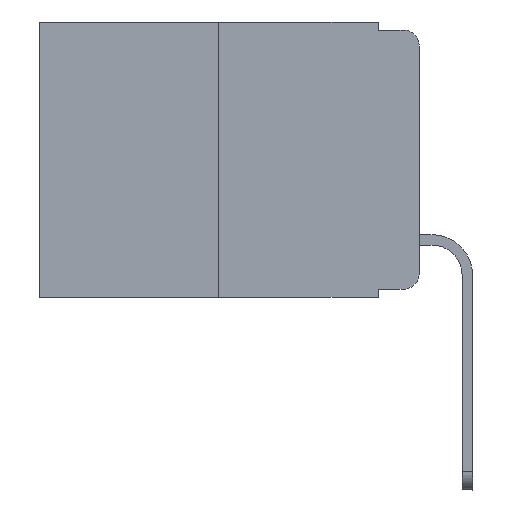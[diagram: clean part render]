
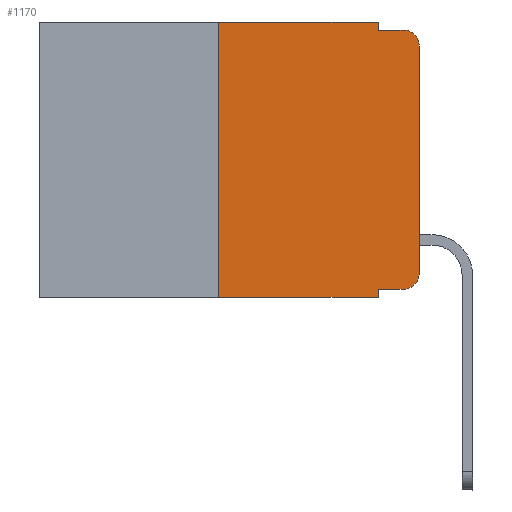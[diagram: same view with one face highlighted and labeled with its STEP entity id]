
A CAD part, left-side view. The second image highlights one B-rep face of the part: STEP entity #1170.
In plain terms, the highlighted planar face has unit normal (-1, 0, 0).
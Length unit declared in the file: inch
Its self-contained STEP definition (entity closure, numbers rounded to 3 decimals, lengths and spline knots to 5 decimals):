
#82 = EDGE_CURVE ( 'NONE', #13693, #13190, #6602, .T. ) ;
#115 = CARTESIAN_POINT ( 'NONE',  ( 0., 0.02, -0.333 ) ) ;
#317 = DIRECTION ( 'NONE',  ( 0., 0., -1. ) ) ;
#333 = DIRECTION ( 'NONE',  ( 0., -1., 0. ) ) ;
#436 = CARTESIAN_POINT ( 'NONE',  ( 0., 0.051, -0.01 ) ) ;
#556 = CARTESIAN_POINT ( 'NONE',  ( 0., 0.25, 0. ) ) ;
#611 = EDGE_CURVE ( 'NONE', #15490, #10977, #10790, .T. ) ;
#653 = CARTESIAN_POINT ( 'NONE',  ( 0., 0.02, -0.01 ) ) ;
#894 = CARTESIAN_POINT ( 'NONE',  ( 0., 0.25, 0. ) ) ;
#1017 = DIRECTION ( 'NONE',  ( -1., 0., 0. ) ) ;
#1170 = ADVANCED_FACE ( 'NONE', ( #13614 ), #2531, .F. ) ;
#1181 = CARTESIAN_POINT ( 'NONE',  ( 0., 0., -0.313 ) ) ;
#1306 = DIRECTION ( 'NONE',  ( 0., 0., -1. ) ) ;
#1359 = ORIENTED_EDGE ( 'NONE', *, *, #6542, .F. ) ;
#1364 = EDGE_CURVE ( 'NONE', #15490, #9146, #10361, .T. ) ;
#1368 = VECTOR ( 'NONE', #1909, 39.37008 ) ;
#1521 = ORIENTED_EDGE ( 'NONE', *, *, #12869, .T. ) ;
#1689 = ORIENTED_EDGE ( 'NONE', *, *, #82, .T. ) ;
#1909 = DIRECTION ( 'NONE',  ( 0., 0., 1. ) ) ;
#2531 = PLANE ( 'NONE',  #5471 ) ;
#2674 = VECTOR ( 'NONE', #6016, 39.37008 ) ;
#2824 = ORIENTED_EDGE ( 'NONE', *, *, #8174, .T. ) ;
#3003 = ORIENTED_EDGE ( 'NONE', *, *, #15130, .F. ) ;
#3035 = VECTOR ( 'NONE', #333, 39.37008 ) ;
#3454 = CARTESIAN_POINT ( 'NONE',  ( 0., 0.051, -0.333 ) ) ;
#3478 = EDGE_LOOP ( 'NONE', ( #1689, #1521, #12750, #9538, #1359, #10038, #15755, #3003, #7293, #2824 ) ) ;
#3645 = CIRCLE ( 'NONE', #8285, 0.02 ) ;
#4524 = VERTEX_POINT ( 'NONE', #653 ) ;
#4682 = CARTESIAN_POINT ( 'NONE',  ( 0., 0.051, 0. ) ) ;
#4893 = DIRECTION ( 'NONE',  ( 0., 0., -1. ) ) ;
#5294 = DIRECTION ( 'NONE',  ( 0., -1., 0. ) ) ;
#5471 = AXIS2_PLACEMENT_3D ( 'NONE', #9723, #9808, #1306 ) ;
#5951 = EDGE_CURVE ( 'NONE', #10041, #4524, #6272, .T. ) ;
#6016 = DIRECTION ( 'NONE',  ( 0., -1., 0. ) ) ;
#6235 = VERTEX_POINT ( 'NONE', #6415 ) ;
#6272 = LINE ( 'NONE', #11203, #13378 ) ;
#6399 = EDGE_CURVE ( 'NONE', #8701, #11235, #15404, .T. ) ;
#6415 = CARTESIAN_POINT ( 'NONE',  ( 0., 0.051, 0. ) ) ;
#6511 = VECTOR ( 'NONE', #7435, 39.37008 ) ;
#6542 = EDGE_CURVE ( 'NONE', #9146, #6235, #15645, .T. ) ;
#6602 = LINE ( 'NONE', #8048, #1368 ) ;
#6678 = DIRECTION ( 'NONE',  ( 0., 0., -1. ) ) ;
#6872 = DIRECTION ( 'NONE',  ( -1., 0., 0. ) ) ;
#7218 = DIRECTION ( 'NONE',  ( 0., -1., 0. ) ) ;
#7260 = VECTOR ( 'NONE', #15635, 39.37008 ) ;
#7293 = ORIENTED_EDGE ( 'NONE', *, *, #6399, .T. ) ;
#7435 = DIRECTION ( 'NONE',  ( 0., 0., -1. ) ) ;
#8048 = CARTESIAN_POINT ( 'NONE',  ( 0., 0., 0. ) ) ;
#8074 = CARTESIAN_POINT ( 'NONE',  ( 0., 0.02, -0.313 ) ) ;
#8104 = AXIS2_PLACEMENT_3D ( 'NONE', #13009, #1017, #4893 ) ;
#8174 = EDGE_CURVE ( 'NONE', #11235, #13693, #3645, .T. ) ;
#8285 = AXIS2_PLACEMENT_3D ( 'NONE', #8074, #6872, #317 ) ;
#8701 = VERTEX_POINT ( 'NONE', #3454 ) ;
#9146 = VERTEX_POINT ( 'NONE', #556 ) ;
#9299 = EDGE_CURVE ( 'NONE', #6235, #10041, #13507, .T. ) ;
#9538 = ORIENTED_EDGE ( 'NONE', *, *, #9299, .F. ) ;
#9649 = CARTESIAN_POINT ( 'NONE',  ( 0., 0.473, -0.343 ) ) ;
#9723 = CARTESIAN_POINT ( 'NONE',  ( 0., 0.473, 0. ) ) ;
#9808 = DIRECTION ( 'NONE',  ( 1., 0., 0. ) ) ;
#10038 = ORIENTED_EDGE ( 'NONE', *, *, #1364, .F. ) ;
#10041 = VERTEX_POINT ( 'NONE', #436 ) ;
#10361 = LINE ( 'NONE', #894, #7260 ) ;
#10654 = CARTESIAN_POINT ( 'NONE',  ( 0., 0.051, -0.343 ) ) ;
#10790 = LINE ( 'NONE', #9649, #2674 ) ;
#10977 = VERTEX_POINT ( 'NONE', #10654 ) ;
#11059 = VECTOR ( 'NONE', #7218, 39.37008 ) ;
#11203 = CARTESIAN_POINT ( 'NONE',  ( 0., 0.051, -0.01 ) ) ;
#11235 = VERTEX_POINT ( 'NONE', #115 ) ;
#11769 = LINE ( 'NONE', #12830, #14652 ) ;
#11989 = CIRCLE ( 'NONE', #8104, 0.02 ) ;
#12216 = CARTESIAN_POINT ( 'NONE',  ( 0., 0., -0.03 ) ) ;
#12721 = CARTESIAN_POINT ( 'NONE',  ( 0., 0.051, -0.333 ) ) ;
#12750 = ORIENTED_EDGE ( 'NONE', *, *, #5951, .F. ) ;
#12830 = CARTESIAN_POINT ( 'NONE',  ( 0., 0.051, 0. ) ) ;
#12869 = EDGE_CURVE ( 'NONE', #13190, #4524, #11989, .T. ) ;
#13009 = CARTESIAN_POINT ( 'NONE',  ( 0., 0.02, -0.03 ) ) ;
#13190 = VERTEX_POINT ( 'NONE', #12216 ) ;
#13378 = VECTOR ( 'NONE', #5294, 39.37008 ) ;
#13507 = LINE ( 'NONE', #4682, #6511 ) ;
#13614 = FACE_OUTER_BOUND ( 'NONE', #3478, .T. ) ;
#13693 = VERTEX_POINT ( 'NONE', #1181 ) ;
#14652 = VECTOR ( 'NONE', #6678, 39.37008 ) ;
#14938 = CARTESIAN_POINT ( 'NONE',  ( 0., 0.25, -0.343 ) ) ;
#15130 = EDGE_CURVE ( 'NONE', #8701, #10977, #11769, .T. ) ;
#15404 = LINE ( 'NONE', #12721, #3035 ) ;
#15490 = VERTEX_POINT ( 'NONE', #14938 ) ;
#15635 = DIRECTION ( 'NONE',  ( 0., 0., 1. ) ) ;
#15645 = LINE ( 'NONE', #15731, #11059 ) ;
#15731 = CARTESIAN_POINT ( 'NONE',  ( 0., 0.473, 0. ) ) ;
#15755 = ORIENTED_EDGE ( 'NONE', *, *, #611, .T. ) ;
